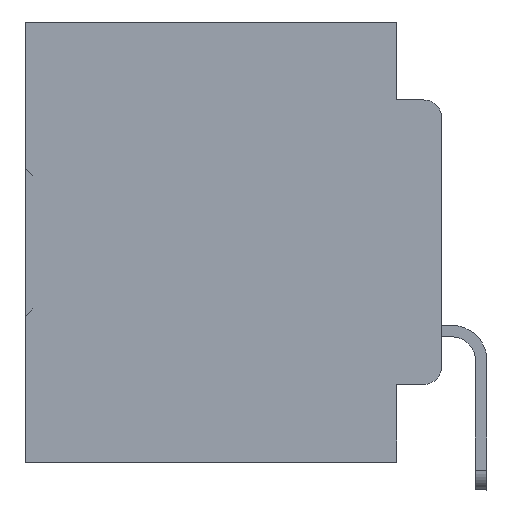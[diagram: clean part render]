
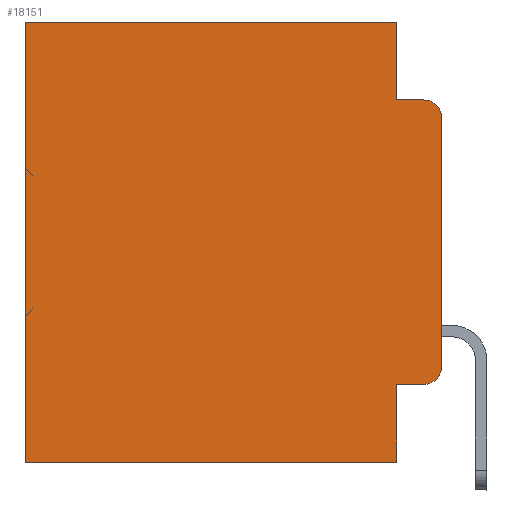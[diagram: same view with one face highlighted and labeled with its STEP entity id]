
A CAD part, left-side view. The second image highlights one B-rep face of the part: STEP entity #18151.
In plain terms, the highlighted planar face has unit normal (-1, 0, 0).
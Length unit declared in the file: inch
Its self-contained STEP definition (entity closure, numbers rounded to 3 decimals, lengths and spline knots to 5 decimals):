
#170 = LINE ( 'NONE', #26276, #20376 ) ;
#558 = DIRECTION ( 'NONE',  ( 0., 1., 0. ) ) ;
#588 = LINE ( 'NONE', #5682, #30312 ) ;
#782 = LINE ( 'NONE', #7062, #29595 ) ;
#953 = VERTEX_POINT ( 'NONE', #10217 ) ;
#1339 = CARTESIAN_POINT ( 'NONE',  ( 0.298, 0.02, -0.1085 ) ) ;
#1423 = ORIENTED_EDGE ( 'NONE', *, *, #35210, .T. ) ;
#1492 = EDGE_CURVE ( 'NONE', #4919, #3664, #20566, .T. ) ;
#1543 = ORIENTED_EDGE ( 'NONE', *, *, #4762, .F. ) ;
#1745 = CARTESIAN_POINT ( 'NONE',  ( 0.298, 0.02, -0.3915 ) ) ;
#1827 = DIRECTION ( 'NONE',  ( 0., -1., 0. ) ) ;
#2464 = LINE ( 'NONE', #30904, #34884 ) ;
#3109 = ORIENTED_EDGE ( 'NONE', *, *, #30452, .F. ) ;
#3116 = ORIENTED_EDGE ( 'NONE', *, *, #8099, .T. ) ;
#3407 = EDGE_CURVE ( 'NONE', #10748, #3664, #11013, .T. ) ;
#3613 = EDGE_CURVE ( 'NONE', #4919, #31343, #33965, .T. ) ;
#3664 = VERTEX_POINT ( 'NONE', #16019 ) ;
#3694 = DIRECTION ( 'NONE',  ( 1., 0., 0. ) ) ;
#3735 = ORIENTED_EDGE ( 'NONE', *, *, #23442, .F. ) ;
#3756 = CARTESIAN_POINT ( 'NONE',  ( 0.298, 0.051, -0.4115 ) ) ;
#4762 = EDGE_CURVE ( 'NONE', #25147, #20265, #782, .T. ) ;
#4919 = VERTEX_POINT ( 'NONE', #28576 ) ;
#5682 = CARTESIAN_POINT ( 'NONE',  ( 0.298, 0.473, 0. ) ) ;
#6111 = CARTESIAN_POINT ( 'NONE',  ( 0.298, 0., -0.5 ) ) ;
#6968 = PLANE ( 'NONE',  #8056 ) ;
#7062 = CARTESIAN_POINT ( 'NONE',  ( 0.298, 0.051, 0. ) ) ;
#7935 = AXIS2_PLACEMENT_3D ( 'NONE', #1745, #24800, #18452 ) ;
#8056 = AXIS2_PLACEMENT_3D ( 'NONE', #17990, #3694, #15360 ) ;
#8099 = EDGE_CURVE ( 'NONE', #9342, #28233, #588, .T. ) ;
#8997 = DIRECTION ( 'NONE',  ( 0., 1., 0. ) ) ;
#9342 = VERTEX_POINT ( 'NONE', #23255 ) ;
#9552 = DIRECTION ( 'NONE',  ( 0., 0., -1. ) ) ;
#10217 = CARTESIAN_POINT ( 'NONE',  ( 0.298, 0.051, 0. ) ) ;
#10748 = VERTEX_POINT ( 'NONE', #21916 ) ;
#10961 = VERTEX_POINT ( 'NONE', #17611 ) ;
#11013 = CIRCLE ( 'NONE', #7935, 0.02 ) ;
#11090 = CARTESIAN_POINT ( 'NONE',  ( 0.298, 0.051, -0.5 ) ) ;
#11498 = DIRECTION ( 'NONE',  ( 0., -1., 0. ) ) ;
#12279 = EDGE_CURVE ( 'NONE', #953, #9342, #170, .T. ) ;
#12449 = FACE_OUTER_BOUND ( 'NONE', #34278, .T. ) ;
#13151 = EDGE_CURVE ( 'NONE', #953, #10961, #36994, .T. ) ;
#13563 = DIRECTION ( 'NONE',  ( 0., 0., -1. ) ) ;
#15314 = ORIENTED_EDGE ( 'NONE', *, *, #13151, .F. ) ;
#15360 = DIRECTION ( 'NONE',  ( 0., 0., -1. ) ) ;
#15855 = AXIS2_PLACEMENT_3D ( 'NONE', #1339, #24641, #18788 ) ;
#16019 = CARTESIAN_POINT ( 'NONE',  ( 0.298, 0., -0.3915 ) ) ;
#16516 = VECTOR ( 'NONE', #11498, 39.37008 ) ;
#17611 = CARTESIAN_POINT ( 'NONE',  ( 0.298, 0.051, -0.0885 ) ) ;
#17990 = CARTESIAN_POINT ( 'NONE',  ( 0.298, 0., 0. ) ) ;
#18151 = ADVANCED_FACE ( 'NONE', ( #12449 ), #6968, .F. ) ;
#18452 = DIRECTION ( 'NONE',  ( 0., 0., -1. ) ) ;
#18788 = DIRECTION ( 'NONE',  ( 0., 0., -1. ) ) ;
#19549 = DIRECTION ( 'NONE',  ( 0., 0., -1. ) ) ;
#19598 = LINE ( 'NONE', #28760, #16516 ) ;
#20265 = VERTEX_POINT ( 'NONE', #11090 ) ;
#20376 = VECTOR ( 'NONE', #8997, 39.37008 ) ;
#20566 = LINE ( 'NONE', #35737, #29188 ) ;
#21916 = CARTESIAN_POINT ( 'NONE',  ( 0.298, 0.02, -0.4115 ) ) ;
#23255 = CARTESIAN_POINT ( 'NONE',  ( 0.298, 0.473, 0. ) ) ;
#23442 = EDGE_CURVE ( 'NONE', #20265, #28233, #35222, .T. ) ;
#23489 = ORIENTED_EDGE ( 'NONE', *, *, #1492, .F. ) ;
#23966 = VECTOR ( 'NONE', #558, 39.37008 ) ;
#24641 = DIRECTION ( 'NONE',  ( -1., 0., 0. ) ) ;
#24800 = DIRECTION ( 'NONE',  ( -1., 0., 0. ) ) ;
#25147 = VERTEX_POINT ( 'NONE', #3756 ) ;
#25430 = DIRECTION ( 'NONE',  ( 0., 0., -1. ) ) ;
#26276 = CARTESIAN_POINT ( 'NONE',  ( 0.298, 0., 0. ) ) ;
#28233 = VERTEX_POINT ( 'NONE', #32484 ) ;
#28576 = CARTESIAN_POINT ( 'NONE',  ( 0.298, 0., -0.1085 ) ) ;
#28760 = CARTESIAN_POINT ( 'NONE',  ( 0.298, 0.051, -0.4115 ) ) ;
#29188 = VECTOR ( 'NONE', #9552, 39.37008 ) ;
#29595 = VECTOR ( 'NONE', #13563, 39.37008 ) ;
#30312 = VECTOR ( 'NONE', #25430, 39.37008 ) ;
#30452 = EDGE_CURVE ( 'NONE', #10961, #31343, #2464, .T. ) ;
#30904 = CARTESIAN_POINT ( 'NONE',  ( 0.298, 0.051, -0.0885 ) ) ;
#31343 = VERTEX_POINT ( 'NONE', #37127 ) ;
#31738 = ORIENTED_EDGE ( 'NONE', *, *, #3407, .T. ) ;
#32484 = CARTESIAN_POINT ( 'NONE',  ( 0.298, 0.473, -0.5 ) ) ;
#32485 = VECTOR ( 'NONE', #19549, 39.37008 ) ;
#33965 = CIRCLE ( 'NONE', #15855, 0.02 ) ;
#34278 = EDGE_LOOP ( 'NONE', ( #23489, #34896, #3109, #15314, #36990, #3116, #3735, #1543, #1423, #31738 ) ) ;
#34884 = VECTOR ( 'NONE', #1827, 39.37008 ) ;
#34896 = ORIENTED_EDGE ( 'NONE', *, *, #3613, .T. ) ;
#35210 = EDGE_CURVE ( 'NONE', #25147, #10748, #19598, .T. ) ;
#35222 = LINE ( 'NONE', #6111, #23966 ) ;
#35737 = CARTESIAN_POINT ( 'NONE',  ( 0.298, 0., 0. ) ) ;
#36990 = ORIENTED_EDGE ( 'NONE', *, *, #12279, .T. ) ;
#36994 = LINE ( 'NONE', #37096, #32485 ) ;
#37096 = CARTESIAN_POINT ( 'NONE',  ( 0.298, 0.051, 0. ) ) ;
#37127 = CARTESIAN_POINT ( 'NONE',  ( 0.298, 0.02, -0.0885 ) ) ;
